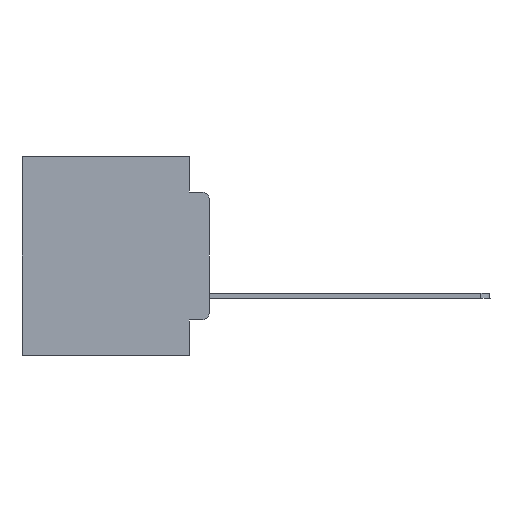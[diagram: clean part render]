
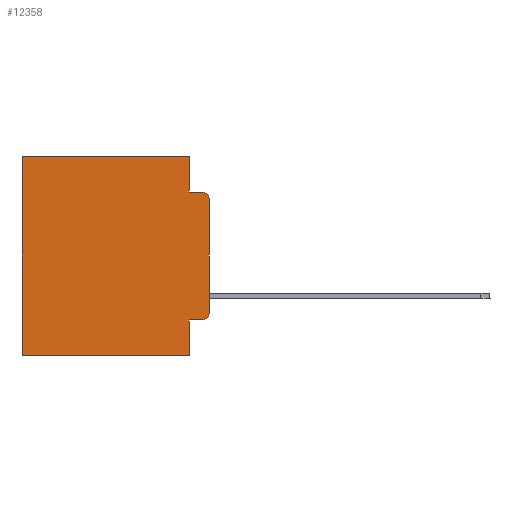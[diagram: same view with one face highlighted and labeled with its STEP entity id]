
A CAD part, left-side view. The second image highlights one B-rep face of the part: STEP entity #12358.
In plain terms, the highlighted planar face has unit normal (-1, 0, 0).
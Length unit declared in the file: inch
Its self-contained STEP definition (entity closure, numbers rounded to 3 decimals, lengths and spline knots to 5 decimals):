
#128 = DIRECTION ( 'NONE',  ( 0., 0., -1. ) ) ;
#373 = LINE ( 'NONE', #4464, #3627 ) ;
#414 = CARTESIAN_POINT ( 'NONE',  ( 0.298, 0., -0.3915 ) ) ;
#771 = LINE ( 'NONE', #13476, #3676 ) ;
#1399 = VERTEX_POINT ( 'NONE', #414 ) ;
#1418 = AXIS2_PLACEMENT_3D ( 'NONE', #12455, #14577, #2123 ) ;
#2123 = DIRECTION ( 'NONE',  ( 0., 0., -1. ) ) ;
#2148 = CARTESIAN_POINT ( 'NONE',  ( 0.298, 0.051, 0. ) ) ;
#2286 = VERTEX_POINT ( 'NONE', #12194 ) ;
#3080 = VERTEX_POINT ( 'NONE', #24035 ) ;
#3361 = DIRECTION ( 'NONE',  ( -1., 0., 0. ) ) ;
#3609 = ORIENTED_EDGE ( 'NONE', *, *, #13443, .F. ) ;
#3627 = VECTOR ( 'NONE', #14912, 39.37008 ) ;
#3676 = VECTOR ( 'NONE', #11385, 39.37008 ) ;
#3955 = LINE ( 'NONE', #23458, #4286 ) ;
#4286 = VECTOR ( 'NONE', #13316, 39.37008 ) ;
#4361 = LINE ( 'NONE', #4725, #8568 ) ;
#4464 = CARTESIAN_POINT ( 'NONE',  ( 0.298, 0.473, 0. ) ) ;
#4712 = VERTEX_POINT ( 'NONE', #25992 ) ;
#4725 = CARTESIAN_POINT ( 'NONE',  ( 0.298, 0.051, -0.0885 ) ) ;
#5994 = CIRCLE ( 'NONE', #8812, 0.02 ) ;
#6292 = PLANE ( 'NONE',  #1418 ) ;
#6386 = DIRECTION ( 'NONE',  ( 0., 0., -1. ) ) ;
#6474 = DIRECTION ( 'NONE',  ( -1., 0., 0. ) ) ;
#6538 = CARTESIAN_POINT ( 'NONE',  ( 0.298, 0.051, -0.4115 ) ) ;
#6748 = EDGE_CURVE ( 'NONE', #12978, #1399, #5994, .T. ) ;
#7157 = CARTESIAN_POINT ( 'NONE',  ( 0.298, 0.051, -0.5 ) ) ;
#7806 = LINE ( 'NONE', #24176, #20437 ) ;
#8568 = VECTOR ( 'NONE', #11507, 39.37008 ) ;
#8736 = VECTOR ( 'NONE', #10722, 39.37008 ) ;
#8812 = AXIS2_PLACEMENT_3D ( 'NONE', #22201, #3361, #9654 ) ;
#9205 = ORIENTED_EDGE ( 'NONE', *, *, #17424, .F. ) ;
#9424 = ORIENTED_EDGE ( 'NONE', *, *, #13647, .T. ) ;
#9466 = VERTEX_POINT ( 'NONE', #20391 ) ;
#9654 = DIRECTION ( 'NONE',  ( 0., 0., -1. ) ) ;
#9761 = ORIENTED_EDGE ( 'NONE', *, *, #24663, .T. ) ;
#10464 = VERTEX_POINT ( 'NONE', #15503 ) ;
#10492 = DIRECTION ( 'NONE',  ( 0., 1., 0. ) ) ;
#10722 = DIRECTION ( 'NONE',  ( 0., -1., 0. ) ) ;
#10861 = EDGE_CURVE ( 'NONE', #4712, #19745, #21879, .T. ) ;
#11385 = DIRECTION ( 'NONE',  ( 0., 1., 0. ) ) ;
#11435 = AXIS2_PLACEMENT_3D ( 'NONE', #12359, #6474, #128 ) ;
#11507 = DIRECTION ( 'NONE',  ( 0., -1., 0. ) ) ;
#11805 = CIRCLE ( 'NONE', #11435, 0.02 ) ;
#12194 = CARTESIAN_POINT ( 'NONE',  ( 0.298, 0.473, 0. ) ) ;
#12358 = ADVANCED_FACE ( 'NONE', ( #17567 ), #6292, .F. ) ;
#12359 = CARTESIAN_POINT ( 'NONE',  ( 0.298, 0.02, -0.1085 ) ) ;
#12455 = CARTESIAN_POINT ( 'NONE',  ( 0.298, 0., 0. ) ) ;
#12513 = EDGE_CURVE ( 'NONE', #18993, #22042, #3955, .T. ) ;
#12662 = CARTESIAN_POINT ( 'NONE',  ( 0.298, 0.02, -0.4115 ) ) ;
#12978 = VERTEX_POINT ( 'NONE', #12662 ) ;
#13316 = DIRECTION ( 'NONE',  ( 0., 0., -1. ) ) ;
#13443 = EDGE_CURVE ( 'NONE', #10464, #1399, #7806, .T. ) ;
#13476 = CARTESIAN_POINT ( 'NONE',  ( 0.298, 0., -0.5 ) ) ;
#13647 = EDGE_CURVE ( 'NONE', #4712, #12978, #14919, .T. ) ;
#14181 = ORIENTED_EDGE ( 'NONE', *, *, #10861, .F. ) ;
#14509 = LINE ( 'NONE', #22772, #24875 ) ;
#14577 = DIRECTION ( 'NONE',  ( 1., 0., 0. ) ) ;
#14912 = DIRECTION ( 'NONE',  ( 0., 0., -1. ) ) ;
#14919 = LINE ( 'NONE', #6538, #8736 ) ;
#14940 = DIRECTION ( 'NONE',  ( 0., 0., -1. ) ) ;
#15452 = EDGE_CURVE ( 'NONE', #18993, #2286, #14509, .T. ) ;
#15503 = CARTESIAN_POINT ( 'NONE',  ( 0.298, 0., -0.1085 ) ) ;
#16238 = ORIENTED_EDGE ( 'NONE', *, *, #23834, .F. ) ;
#17424 = EDGE_CURVE ( 'NONE', #22042, #9466, #4361, .T. ) ;
#17567 = FACE_OUTER_BOUND ( 'NONE', #19729, .T. ) ;
#18002 = EDGE_CURVE ( 'NONE', #10464, #9466, #11805, .T. ) ;
#18314 = VECTOR ( 'NONE', #14940, 39.37008 ) ;
#18676 = CARTESIAN_POINT ( 'NONE',  ( 0.298, 0.051, 0. ) ) ;
#18939 = ORIENTED_EDGE ( 'NONE', *, *, #18002, .T. ) ;
#18993 = VERTEX_POINT ( 'NONE', #18676 ) ;
#19729 = EDGE_LOOP ( 'NONE', ( #3609, #18939, #9205, #24844, #22356, #9761, #16238, #14181, #9424, #23152 ) ) ;
#19745 = VERTEX_POINT ( 'NONE', #7157 ) ;
#20391 = CARTESIAN_POINT ( 'NONE',  ( 0.298, 0.02, -0.0885 ) ) ;
#20437 = VECTOR ( 'NONE', #6386, 39.37008 ) ;
#21879 = LINE ( 'NONE', #2148, #18314 ) ;
#22042 = VERTEX_POINT ( 'NONE', #23457 ) ;
#22201 = CARTESIAN_POINT ( 'NONE',  ( 0.298, 0.02, -0.3915 ) ) ;
#22356 = ORIENTED_EDGE ( 'NONE', *, *, #15452, .T. ) ;
#22772 = CARTESIAN_POINT ( 'NONE',  ( 0.298, 0., 0. ) ) ;
#23152 = ORIENTED_EDGE ( 'NONE', *, *, #6748, .T. ) ;
#23457 = CARTESIAN_POINT ( 'NONE',  ( 0.298, 0.051, -0.0885 ) ) ;
#23458 = CARTESIAN_POINT ( 'NONE',  ( 0.298, 0.051, 0. ) ) ;
#23834 = EDGE_CURVE ( 'NONE', #19745, #3080, #771, .T. ) ;
#24035 = CARTESIAN_POINT ( 'NONE',  ( 0.298, 0.473, -0.5 ) ) ;
#24176 = CARTESIAN_POINT ( 'NONE',  ( 0.298, 0., 0. ) ) ;
#24663 = EDGE_CURVE ( 'NONE', #2286, #3080, #373, .T. ) ;
#24844 = ORIENTED_EDGE ( 'NONE', *, *, #12513, .F. ) ;
#24875 = VECTOR ( 'NONE', #10492, 39.37008 ) ;
#25992 = CARTESIAN_POINT ( 'NONE',  ( 0.298, 0.051, -0.4115 ) ) ;
